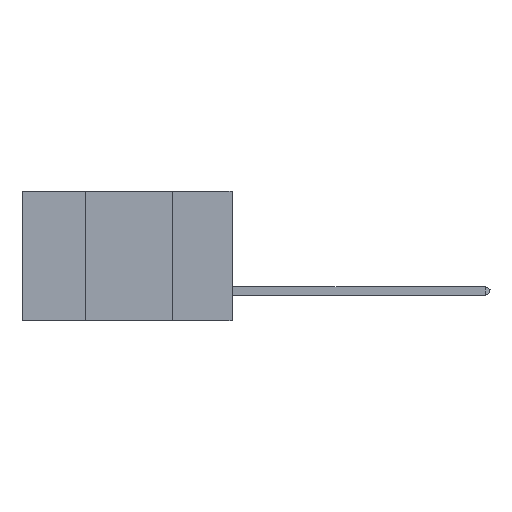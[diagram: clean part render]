
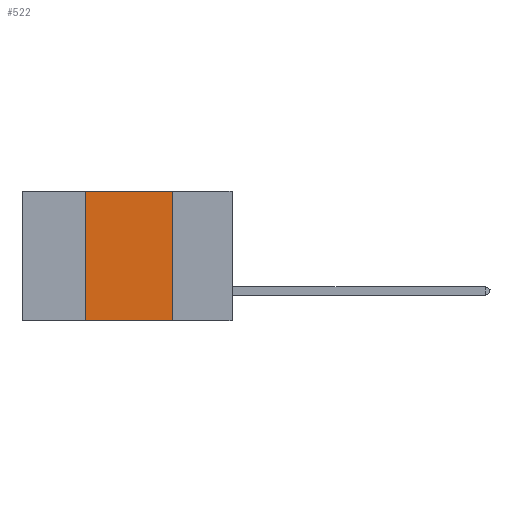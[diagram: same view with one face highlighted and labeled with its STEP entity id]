
A CAD part, left-side view. The second image highlights one B-rep face of the part: STEP entity #522.
In plain terms, the highlighted planar face has unit normal (-1, 0, 0).
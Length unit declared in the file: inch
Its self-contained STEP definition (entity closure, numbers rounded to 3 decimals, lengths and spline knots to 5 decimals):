
#426 = ORIENTED_EDGE ( 'NONE', *, *, #31790, .F. ) ;
#475 = CARTESIAN_POINT ( 'NONE',  ( 0., 0.6, -0.37 ) ) ;
#522 = ADVANCED_FACE ( 'NONE', ( #21789 ), #17658, .F. ) ;
#629 = DIRECTION ( 'NONE',  ( 0., -1., 0. ) ) ;
#2701 = VECTOR ( 'NONE', #629, 39.37008 ) ;
#4418 = DIRECTION ( 'NONE',  ( 0., 0., -1. ) ) ;
#4457 = VECTOR ( 'NONE', #13192, 39.37008 ) ;
#4992 = CARTESIAN_POINT ( 'NONE',  ( 0., 0.42, 0. ) ) ;
#5630 = CARTESIAN_POINT ( 'NONE',  ( 0., 0.42, 0. ) ) ;
#5688 = EDGE_CURVE ( 'NONE', #38807, #29697, #40440, .T. ) ;
#6099 = LINE ( 'NONE', #41373, #24886 ) ;
#6212 = CARTESIAN_POINT ( 'NONE',  ( 0., 0.17, 0. ) ) ;
#6519 = VERTEX_POINT ( 'NONE', #39841 ) ;
#8414 = LINE ( 'NONE', #475, #2701 ) ;
#9588 = VECTOR ( 'NONE', #39043, 39.37008 ) ;
#12043 = ORIENTED_EDGE ( 'NONE', *, *, #39476, .T. ) ;
#13192 = DIRECTION ( 'NONE',  ( 0., 0., -1. ) ) ;
#14127 = EDGE_CURVE ( 'NONE', #6519, #39660, #23184, .T. ) ;
#14536 = ORIENTED_EDGE ( 'NONE', *, *, #5688, .F. ) ;
#17658 = PLANE ( 'NONE',  #20177 ) ;
#17943 = CARTESIAN_POINT ( 'NONE',  ( 0., 0.6, 0. ) ) ;
#19183 = CARTESIAN_POINT ( 'NONE',  ( 0., 0.17, -0.37 ) ) ;
#20177 = AXIS2_PLACEMENT_3D ( 'NONE', #17943, #27492, #4418 ) ;
#21339 = DIRECTION ( 'NONE',  ( 0., -1., 0. ) ) ;
#21789 = FACE_OUTER_BOUND ( 'NONE', #43084, .T. ) ;
#23184 = LINE ( 'NONE', #5630, #9588 ) ;
#24886 = VECTOR ( 'NONE', #21339, 39.37008 ) ;
#25996 = ORIENTED_EDGE ( 'NONE', *, *, #14127, .F. ) ;
#26350 = CARTESIAN_POINT ( 'NONE',  ( 0., 0.17, 0. ) ) ;
#27492 = DIRECTION ( 'NONE',  ( 1., 0., 0. ) ) ;
#29697 = VERTEX_POINT ( 'NONE', #19183 ) ;
#31790 = EDGE_CURVE ( 'NONE', #39660, #38807, #6099, .T. ) ;
#38807 = VERTEX_POINT ( 'NONE', #6212 ) ;
#39043 = DIRECTION ( 'NONE',  ( 0., 0., 1. ) ) ;
#39476 = EDGE_CURVE ( 'NONE', #6519, #29697, #8414, .T. ) ;
#39660 = VERTEX_POINT ( 'NONE', #4992 ) ;
#39841 = CARTESIAN_POINT ( 'NONE',  ( 0., 0.42, -0.37 ) ) ;
#40440 = LINE ( 'NONE', #26350, #4457 ) ;
#41373 = CARTESIAN_POINT ( 'NONE',  ( 0., 0.6, 0. ) ) ;
#43084 = EDGE_LOOP ( 'NONE', ( #14536, #426, #25996, #12043 ) ) ;
